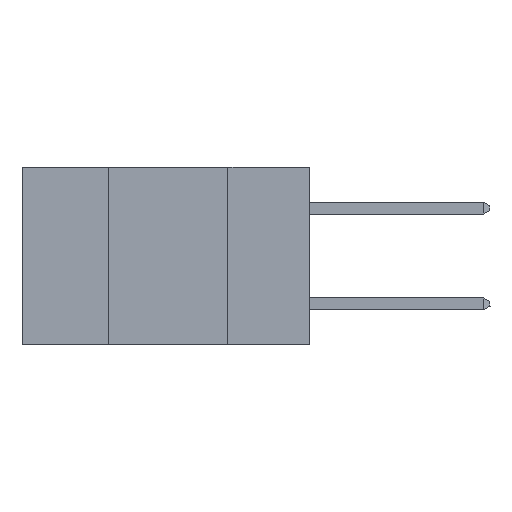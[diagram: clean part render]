
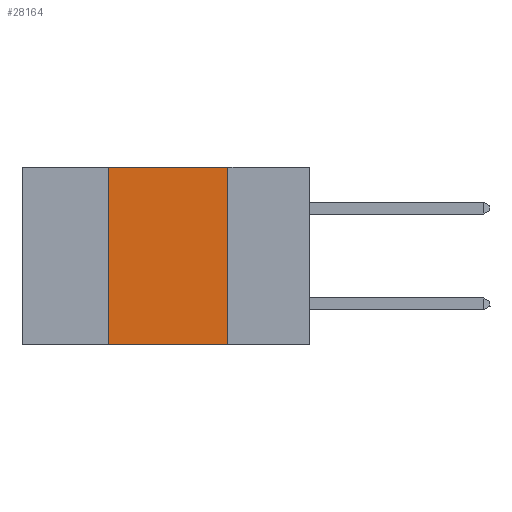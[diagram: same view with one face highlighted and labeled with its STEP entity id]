
A CAD part, left-side view. The second image highlights one B-rep face of the part: STEP entity #28164.
In plain terms, the highlighted planar face has unit normal (-1, 0, 0).
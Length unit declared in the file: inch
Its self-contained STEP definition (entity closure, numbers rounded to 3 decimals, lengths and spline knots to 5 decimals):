
#2258 = VECTOR ( 'NONE', #7443, 39.37008 ) ;
#3233 = AXIS2_PLACEMENT_3D ( 'NONE', #5853, #27301, #3498 ) ;
#3498 = DIRECTION ( 'NONE',  ( 0., 0., -1. ) ) ;
#4505 = CARTESIAN_POINT ( 'NONE',  ( 0., 0.42, 0. ) ) ;
#5203 = CARTESIAN_POINT ( 'NONE',  ( 0., 0.6, -0.37 ) ) ;
#5723 = CARTESIAN_POINT ( 'NONE',  ( 0., 0.42, 0. ) ) ;
#5733 = CARTESIAN_POINT ( 'NONE',  ( 0., 0.17, -0.37 ) ) ;
#5853 = CARTESIAN_POINT ( 'NONE',  ( 0., 0.6, 0. ) ) ;
#6280 = EDGE_CURVE ( 'NONE', #13611, #12057, #28135, .T. ) ;
#7443 = DIRECTION ( 'NONE',  ( 0., -1., 0. ) ) ;
#8209 = PLANE ( 'NONE',  #3233 ) ;
#9196 = DIRECTION ( 'NONE',  ( 0., 0., 1. ) ) ;
#9482 = CARTESIAN_POINT ( 'NONE',  ( 0., 0.6, 0. ) ) ;
#10416 = ORIENTED_EDGE ( 'NONE', *, *, #29326, .F. ) ;
#10693 = VECTOR ( 'NONE', #9196, 39.37008 ) ;
#12057 = VERTEX_POINT ( 'NONE', #5723 ) ;
#13611 = VERTEX_POINT ( 'NONE', #28890 ) ;
#17091 = VECTOR ( 'NONE', #21504, 39.37008 ) ;
#18111 = EDGE_CURVE ( 'NONE', #13611, #22755, #21340, .T. ) ;
#18980 = ORIENTED_EDGE ( 'NONE', *, *, #25552, .F. ) ;
#19064 = VERTEX_POINT ( 'NONE', #25680 ) ;
#20233 = VECTOR ( 'NONE', #22501, 39.37008 ) ;
#21340 = LINE ( 'NONE', #5203, #17091 ) ;
#21504 = DIRECTION ( 'NONE',  ( 0., -1., 0. ) ) ;
#22274 = ORIENTED_EDGE ( 'NONE', *, *, #6280, .F. ) ;
#22501 = DIRECTION ( 'NONE',  ( 0., 0., -1. ) ) ;
#22755 = VERTEX_POINT ( 'NONE', #5733 ) ;
#22995 = EDGE_LOOP ( 'NONE', ( #18980, #10416, #22274, #26699 ) ) ;
#24840 = LINE ( 'NONE', #27646, #20233 ) ;
#25552 = EDGE_CURVE ( 'NONE', #19064, #22755, #24840, .T. ) ;
#25680 = CARTESIAN_POINT ( 'NONE',  ( 0., 0.17, 0. ) ) ;
#26699 = ORIENTED_EDGE ( 'NONE', *, *, #18111, .T. ) ;
#27301 = DIRECTION ( 'NONE',  ( 1., 0., 0. ) ) ;
#27646 = CARTESIAN_POINT ( 'NONE',  ( 0., 0.17, 0. ) ) ;
#28135 = LINE ( 'NONE', #4505, #10693 ) ;
#28164 = ADVANCED_FACE ( 'NONE', ( #29795 ), #8209, .F. ) ;
#28720 = LINE ( 'NONE', #9482, #2258 ) ;
#28890 = CARTESIAN_POINT ( 'NONE',  ( 0., 0.42, -0.37 ) ) ;
#29326 = EDGE_CURVE ( 'NONE', #12057, #19064, #28720, .T. ) ;
#29795 = FACE_OUTER_BOUND ( 'NONE', #22995, .T. ) ;
